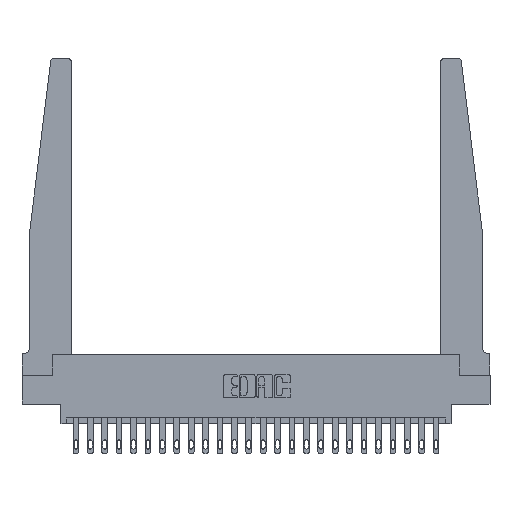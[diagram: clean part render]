
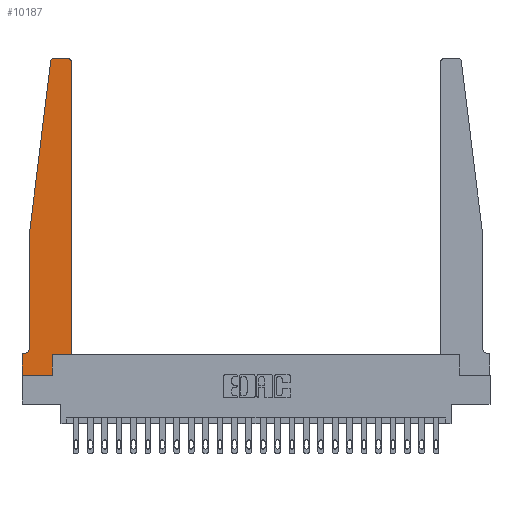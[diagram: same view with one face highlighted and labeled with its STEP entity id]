
A CAD part, top view. The second image highlights one B-rep face of the part: STEP entity #10187.
In plain terms, the highlighted planar face has unit normal (0, 0, 1).
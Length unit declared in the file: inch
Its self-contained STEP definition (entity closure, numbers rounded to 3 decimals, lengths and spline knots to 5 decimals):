
#75 = DIRECTION ( 'NONE',  ( 0., 1., 0. ) ) ;
#499 = CARTESIAN_POINT ( 'NONE',  ( 0.395, 2.75, 0.37 ) ) ;
#692 = EDGE_CURVE ( 'NONE', #5523, #5949, #20826, .T. ) ;
#711 = LINE ( 'NONE', #8235, #19833 ) ;
#831 = VERTEX_POINT ( 'NONE', #23151 ) ;
#998 = ORIENTED_EDGE ( 'NONE', *, *, #12638, .T. ) ;
#1186 = VECTOR ( 'NONE', #6332, 39.37008 ) ;
#1189 = ORIENTED_EDGE ( 'NONE', *, *, #17300, .T. ) ;
#1317 = CARTESIAN_POINT ( 'NONE',  ( 0.065, 0.1875, 0.37 ) ) ;
#1436 = ORIENTED_EDGE ( 'NONE', *, *, #3732, .T. ) ;
#2002 = EDGE_CURVE ( 'NONE', #21255, #19215, #12724, .T. ) ;
#2814 = CARTESIAN_POINT ( 'NONE',  ( 0.425, 0.18, 0.37 ) ) ;
#3732 = EDGE_CURVE ( 'NONE', #7690, #831, #19870, .T. ) ;
#3956 = EDGE_LOOP ( 'NONE', ( #14498, #8123, #1436, #19125, #12263, #13855, #5236, #23296, #18875, #1189, #10777, #998 ) ) ;
#4549 = DIRECTION ( 'NONE',  ( 0., 0., -1. ) ) ;
#4971 = VECTOR ( 'NONE', #5075, 39.37008 ) ;
#5044 = VECTOR ( 'NONE', #75, 39.37008 ) ;
#5073 = CARTESIAN_POINT ( 'NONE',  ( 0.27653, 2.75, 0.37 ) ) ;
#5075 = DIRECTION ( 'NONE',  ( -1., 0., 0. ) ) ;
#5231 = CIRCLE ( 'NONE', #8414, 0.05 ) ;
#5236 = ORIENTED_EDGE ( 'NONE', *, *, #11475, .T. ) ;
#5323 = EDGE_CURVE ( 'NONE', #831, #24182, #711, .T. ) ;
#5485 = CARTESIAN_POINT ( 'NONE',  ( 0.2605, 0.18, 0.37 ) ) ;
#5523 = VERTEX_POINT ( 'NONE', #13708 ) ;
#5949 = VERTEX_POINT ( 'NONE', #20447 ) ;
#6013 = CARTESIAN_POINT ( 'NONE',  ( 0.065, 0.2375, 0.37 ) ) ;
#6332 = DIRECTION ( 'NONE',  ( 1., 0., 0. ) ) ;
#6832 = AXIS2_PLACEMENT_3D ( 'NONE', #10863, #22062, #20109 ) ;
#7237 = CARTESIAN_POINT ( 'NONE',  ( 0.425, 2.72, 0.37 ) ) ;
#7671 = VECTOR ( 'NONE', #14380, 39.37008 ) ;
#7690 = VERTEX_POINT ( 'NONE', #8406 ) ;
#7967 = DIRECTION ( 'NONE',  ( 0., 0., 1. ) ) ;
#7987 = DIRECTION ( 'NONE',  ( 0., -1., 0. ) ) ;
#8123 = ORIENTED_EDGE ( 'NONE', *, *, #19755, .T. ) ;
#8235 = CARTESIAN_POINT ( 'NONE',  ( 0.065, 1.25, 0.37 ) ) ;
#8406 = CARTESIAN_POINT ( 'NONE',  ( 0.24675, 2.72367, 0.37 ) ) ;
#8414 = AXIS2_PLACEMENT_3D ( 'NONE', #23474, #4549, #21616 ) ;
#8562 = CARTESIAN_POINT ( 'NONE',  ( 0.25, 2.75, 0.37 ) ) ;
#8928 = CIRCLE ( 'NONE', #19284, 0.03 ) ;
#8989 = LINE ( 'NONE', #10636, #21568 ) ;
#9929 = CARTESIAN_POINT ( 'NONE',  ( 0.425, 0.18, 0.37 ) ) ;
#10187 = ADVANCED_FACE ( 'NONE', ( #18493 ), #10749, .T. ) ;
#10522 = LINE ( 'NONE', #2814, #21825 ) ;
#10636 = CARTESIAN_POINT ( 'NONE',  ( 0., 0., 0.37 ) ) ;
#10749 = PLANE ( 'NONE',  #6832 ) ;
#10777 = ORIENTED_EDGE ( 'NONE', *, *, #22712, .T. ) ;
#10863 = CARTESIAN_POINT ( 'NONE',  ( 0., 0.1875, 0.37 ) ) ;
#10986 = DIRECTION ( 'NONE',  ( 0., -1., 0. ) ) ;
#11475 = EDGE_CURVE ( 'NONE', #19215, #22713, #8989, .T. ) ;
#12199 = VERTEX_POINT ( 'NONE', #15647 ) ;
#12263 = ORIENTED_EDGE ( 'NONE', *, *, #16653, .T. ) ;
#12375 = DIRECTION ( 'NONE',  ( 1., 0., 0. ) ) ;
#12387 = DIRECTION ( 'NONE',  ( 0., 1., 0. ) ) ;
#12633 = LINE ( 'NONE', #17913, #7671 ) ;
#12638 = EDGE_CURVE ( 'NONE', #19506, #20559, #12804, .T. ) ;
#12724 = LINE ( 'NONE', #1317, #13834 ) ;
#12804 = CIRCLE ( 'NONE', #20662, 0.03 ) ;
#13708 = CARTESIAN_POINT ( 'NONE',  ( 0.2605, 0., 0.37 ) ) ;
#13834 = VECTOR ( 'NONE', #21953, 39.37008 ) ;
#13855 = ORIENTED_EDGE ( 'NONE', *, *, #2002, .T. ) ;
#14380 = DIRECTION ( 'NONE',  ( 1., 0., 0. ) ) ;
#14483 = DIRECTION ( 'NONE',  ( -0.122, -0.992, 0. ) ) ;
#14498 = ORIENTED_EDGE ( 'NONE', *, *, #21563, .T. ) ;
#15647 = CARTESIAN_POINT ( 'NONE',  ( 0.425, 0.18, 0.37 ) ) ;
#15664 = CARTESIAN_POINT ( 'NONE',  ( 0.27653, 2.72, 0.37 ) ) ;
#16204 = CARTESIAN_POINT ( 'NONE',  ( 0.395, 2.72, 0.37 ) ) ;
#16270 = VERTEX_POINT ( 'NONE', #5073 ) ;
#16653 = EDGE_CURVE ( 'NONE', #24182, #21255, #5231, .T. ) ;
#17300 = EDGE_CURVE ( 'NONE', #5949, #12199, #23263, .T. ) ;
#17830 = LINE ( 'NONE', #8562, #4971 ) ;
#17913 = CARTESIAN_POINT ( 'NONE',  ( 0., 0., 0.37 ) ) ;
#18493 = FACE_OUTER_BOUND ( 'NONE', #3956, .T. ) ;
#18715 = CARTESIAN_POINT ( 'NONE',  ( 0.065, 1.25, 0.37 ) ) ;
#18875 = ORIENTED_EDGE ( 'NONE', *, *, #692, .T. ) ;
#19125 = ORIENTED_EDGE ( 'NONE', *, *, #5323, .T. ) ;
#19206 = DIRECTION ( 'NONE',  ( 1., 0., 0. ) ) ;
#19215 = VERTEX_POINT ( 'NONE', #21097 ) ;
#19284 = AXIS2_PLACEMENT_3D ( 'NONE', #15664, #7967, #19206 ) ;
#19506 = VERTEX_POINT ( 'NONE', #7237 ) ;
#19755 = EDGE_CURVE ( 'NONE', #16270, #7690, #8928, .T. ) ;
#19833 = VECTOR ( 'NONE', #7987, 39.37008 ) ;
#19870 = LINE ( 'NONE', #18715, #22108 ) ;
#20109 = DIRECTION ( 'NONE',  ( 1., 0., 0. ) ) ;
#20447 = CARTESIAN_POINT ( 'NONE',  ( 0.2605, 0.18, 0.37 ) ) ;
#20559 = VERTEX_POINT ( 'NONE', #499 ) ;
#20662 = AXIS2_PLACEMENT_3D ( 'NONE', #16204, #23455, #12375 ) ;
#20826 = LINE ( 'NONE', #5485, #5044 ) ;
#21097 = CARTESIAN_POINT ( 'NONE',  ( 0., 0.1875, 0.37 ) ) ;
#21255 = VERTEX_POINT ( 'NONE', #22278 ) ;
#21563 = EDGE_CURVE ( 'NONE', #20559, #16270, #17830, .T. ) ;
#21568 = VECTOR ( 'NONE', #10986, 39.37008 ) ;
#21616 = DIRECTION ( 'NONE',  ( -1., 0., 0. ) ) ;
#21825 = VECTOR ( 'NONE', #12387, 39.37008 ) ;
#21953 = DIRECTION ( 'NONE',  ( -1., 0., 0. ) ) ;
#22062 = DIRECTION ( 'NONE',  ( 0., 0., 1. ) ) ;
#22108 = VECTOR ( 'NONE', #14483, 39.37008 ) ;
#22278 = CARTESIAN_POINT ( 'NONE',  ( 0.015, 0.1875, 0.37 ) ) ;
#22298 = CARTESIAN_POINT ( 'NONE',  ( 0., 0., 0.37 ) ) ;
#22712 = EDGE_CURVE ( 'NONE', #12199, #19506, #10522, .T. ) ;
#22713 = VERTEX_POINT ( 'NONE', #22298 ) ;
#23151 = CARTESIAN_POINT ( 'NONE',  ( 0.065, 1.25, 0.37 ) ) ;
#23263 = LINE ( 'NONE', #9929, #1186 ) ;
#23296 = ORIENTED_EDGE ( 'NONE', *, *, #23920, .T. ) ;
#23455 = DIRECTION ( 'NONE',  ( 0., 0., 1. ) ) ;
#23474 = CARTESIAN_POINT ( 'NONE',  ( 0.015, 0.2375, 0.37 ) ) ;
#23920 = EDGE_CURVE ( 'NONE', #22713, #5523, #12633, .T. ) ;
#24182 = VERTEX_POINT ( 'NONE', #6013 ) ;
